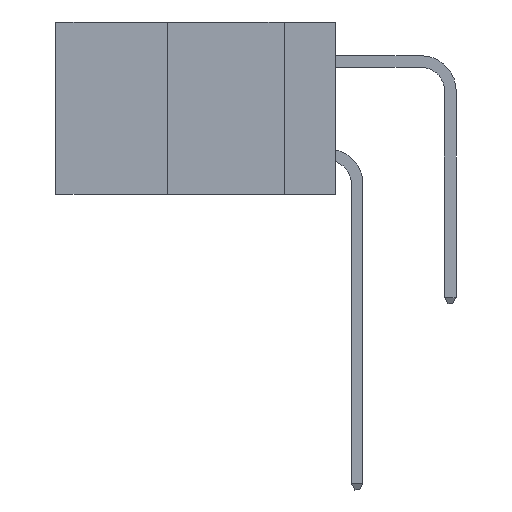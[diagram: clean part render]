
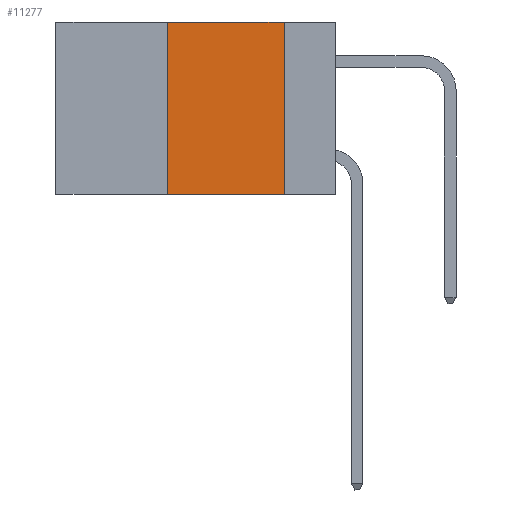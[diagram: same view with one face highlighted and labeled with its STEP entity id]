
A CAD part, left-side view. The second image highlights one B-rep face of the part: STEP entity #11277.
In plain terms, the highlighted planar face has unit normal (-1, 0, 0).
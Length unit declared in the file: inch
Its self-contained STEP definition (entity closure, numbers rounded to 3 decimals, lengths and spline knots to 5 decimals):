
#770 = LINE ( 'NONE', #20376, #15443 ) ;
#1799 = CARTESIAN_POINT ( 'NONE',  ( 0., 0.36, 0. ) ) ;
#2462 = CARTESIAN_POINT ( 'NONE',  ( 0., 0.6, 0. ) ) ;
#3764 = VERTEX_POINT ( 'NONE', #5386 ) ;
#3811 = EDGE_CURVE ( 'NONE', #3764, #19587, #770, .T. ) ;
#4407 = DIRECTION ( 'NONE',  ( 1., 0., 0. ) ) ;
#5386 = CARTESIAN_POINT ( 'NONE',  ( 0., 0.11, 0. ) ) ;
#5971 = CARTESIAN_POINT ( 'NONE',  ( 0., 0.6, 0. ) ) ;
#7488 = VECTOR ( 'NONE', #20403, 39.37008 ) ;
#7897 = DIRECTION ( 'NONE',  ( 0., -1., 0. ) ) ;
#7984 = VERTEX_POINT ( 'NONE', #1799 ) ;
#8978 = LINE ( 'NONE', #5971, #23082 ) ;
#9240 = EDGE_LOOP ( 'NONE', ( #23718, #15276, #10863, #16390 ) ) ;
#9306 = DIRECTION ( 'NONE',  ( 0., 0., -1. ) ) ;
#10706 = CARTESIAN_POINT ( 'NONE',  ( 0., 0.11, -0.37 ) ) ;
#10863 = ORIENTED_EDGE ( 'NONE', *, *, #16047, .F. ) ;
#11024 = EDGE_CURVE ( 'NONE', #15781, #19587, #13154, .T. ) ;
#11277 = ADVANCED_FACE ( 'NONE', ( #11668 ), #13877, .F. ) ;
#11636 = DIRECTION ( 'NONE',  ( 0., 0., 1. ) ) ;
#11668 = FACE_OUTER_BOUND ( 'NONE', #9240, .T. ) ;
#13154 = LINE ( 'NONE', #15043, #7488 ) ;
#13877 = PLANE ( 'NONE',  #16719 ) ;
#15043 = CARTESIAN_POINT ( 'NONE',  ( 0., 0.6, -0.37 ) ) ;
#15276 = ORIENTED_EDGE ( 'NONE', *, *, #22524, .F. ) ;
#15443 = VECTOR ( 'NONE', #9306, 39.37008 ) ;
#15781 = VERTEX_POINT ( 'NONE', #16349 ) ;
#16047 = EDGE_CURVE ( 'NONE', #15781, #7984, #24254, .T. ) ;
#16349 = CARTESIAN_POINT ( 'NONE',  ( 0., 0.36, -0.37 ) ) ;
#16390 = ORIENTED_EDGE ( 'NONE', *, *, #11024, .T. ) ;
#16719 = AXIS2_PLACEMENT_3D ( 'NONE', #2462, #4407, #17563 ) ;
#17563 = DIRECTION ( 'NONE',  ( 0., 0., -1. ) ) ;
#19587 = VERTEX_POINT ( 'NONE', #10706 ) ;
#20376 = CARTESIAN_POINT ( 'NONE',  ( 0., 0.11, 0. ) ) ;
#20403 = DIRECTION ( 'NONE',  ( 0., -1., 0. ) ) ;
#21714 = VECTOR ( 'NONE', #11636, 39.37008 ) ;
#22524 = EDGE_CURVE ( 'NONE', #7984, #3764, #8978, .T. ) ;
#22548 = CARTESIAN_POINT ( 'NONE',  ( 0., 0.36, 0. ) ) ;
#23082 = VECTOR ( 'NONE', #7897, 39.37008 ) ;
#23718 = ORIENTED_EDGE ( 'NONE', *, *, #3811, .F. ) ;
#24254 = LINE ( 'NONE', #22548, #21714 ) ;
